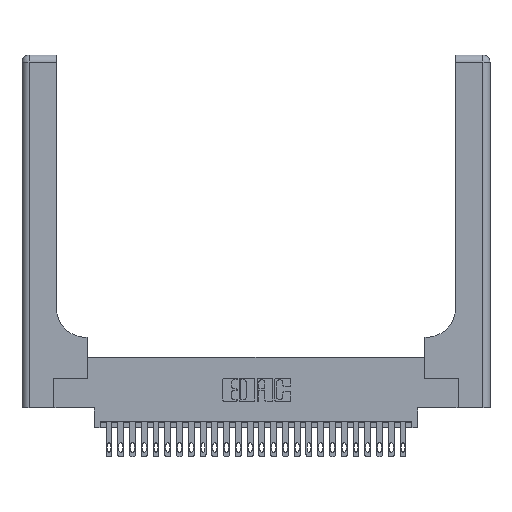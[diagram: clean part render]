
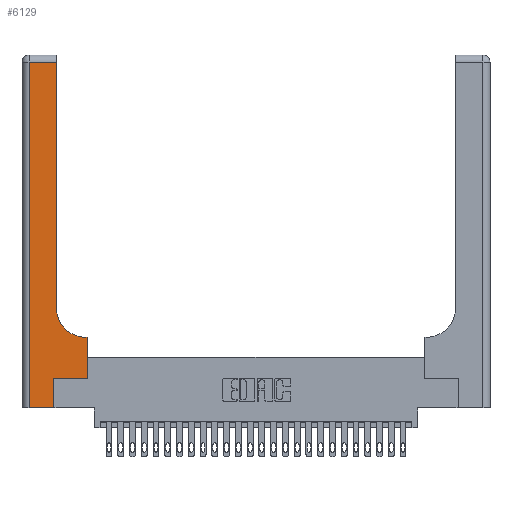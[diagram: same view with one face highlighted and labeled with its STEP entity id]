
A CAD part, top view. The second image highlights one B-rep face of the part: STEP entity #6129.
In plain terms, the highlighted planar face has unit normal (0, 0, 1).
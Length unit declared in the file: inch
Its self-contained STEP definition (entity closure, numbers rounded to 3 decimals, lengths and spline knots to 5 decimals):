
#206 = LINE ( 'NONE', #2875, #23415 ) ;
#1153 = ORIENTED_EDGE ( 'NONE', *, *, #12919, .T. ) ;
#1300 = DIRECTION ( 'NONE',  ( 0., 1., 0. ) ) ;
#1729 = CARTESIAN_POINT ( 'NONE',  ( 0.5585, 0.25, 0.37 ) ) ;
#2001 = CARTESIAN_POINT ( 'NONE',  ( 0.06, 0., 0.37 ) ) ;
#2509 = VERTEX_POINT ( 'NONE', #13331 ) ;
#2572 = LINE ( 'NONE', #18681, #14012 ) ;
#2723 = DIRECTION ( 'NONE',  ( 1., 0., 0. ) ) ;
#2875 = CARTESIAN_POINT ( 'NONE',  ( 0.2915, 3., 0.37 ) ) ;
#3445 = VERTEX_POINT ( 'NONE', #1729 ) ;
#3664 = VERTEX_POINT ( 'NONE', #20395 ) ;
#3770 = VERTEX_POINT ( 'NONE', #18522 ) ;
#4890 = DIRECTION ( 'NONE',  ( -1., 0., 0. ) ) ;
#5336 = EDGE_CURVE ( 'NONE', #13133, #3445, #2572, .T. ) ;
#5775 = EDGE_CURVE ( 'NONE', #22903, #21329, #206, .T. ) ;
#6126 = CARTESIAN_POINT ( 'NONE',  ( 0.2915, 0.6, 0.37 ) ) ;
#6129 = ADVANCED_FACE ( 'NONE', ( #10603 ), #26612, .F. ) ;
#6172 = EDGE_CURVE ( 'NONE', #3664, #22903, #14320, .T. ) ;
#6247 = EDGE_CURVE ( 'NONE', #21329, #3770, #11279, .T. ) ;
#6264 = DIRECTION ( 'NONE',  ( 1., 0., 0. ) ) ;
#6644 = DIRECTION ( 'NONE',  ( 0., -1., 0. ) ) ;
#6783 = LINE ( 'NONE', #12752, #20249 ) ;
#7349 = ORIENTED_EDGE ( 'NONE', *, *, #21374, .T. ) ;
#7609 = AXIS2_PLACEMENT_3D ( 'NONE', #15793, #13718, #2723 ) ;
#8095 = VECTOR ( 'NONE', #6264, 39.37008 ) ;
#8389 = CARTESIAN_POINT ( 'NONE',  ( 0.269, 0.25, 0.37 ) ) ;
#9195 = LINE ( 'NONE', #12284, #16969 ) ;
#9282 = DIRECTION ( 'NONE',  ( 0., 0., -1. ) ) ;
#9646 = ORIENTED_EDGE ( 'NONE', *, *, #5775, .T. ) ;
#10028 = ORIENTED_EDGE ( 'NONE', *, *, #19236, .T. ) ;
#10079 = EDGE_LOOP ( 'NONE', ( #9646, #27332, #13365, #10028, #1153, #11201, #26944, #7349, #20154 ) ) ;
#10603 = FACE_OUTER_BOUND ( 'NONE', #10079, .T. ) ;
#11201 = ORIENTED_EDGE ( 'NONE', *, *, #5336, .T. ) ;
#11279 = LINE ( 'NONE', #13336, #25764 ) ;
#12284 = CARTESIAN_POINT ( 'NONE',  ( 0.5585, 0.25, 0.37 ) ) ;
#12652 = DIRECTION ( 'NONE',  ( 0., 1., 0. ) ) ;
#12752 = CARTESIAN_POINT ( 'NONE',  ( 0.06, 3., 0.37 ) ) ;
#12919 = EDGE_CURVE ( 'NONE', #16148, #13133, #25143, .T. ) ;
#13133 = VERTEX_POINT ( 'NONE', #8389 ) ;
#13331 = CARTESIAN_POINT ( 'NONE',  ( 0.5585, 0.6, 0.37 ) ) ;
#13336 = CARTESIAN_POINT ( 'NONE',  ( 0., 2.94, 0.37 ) ) ;
#13365 = ORIENTED_EDGE ( 'NONE', *, *, #18548, .T. ) ;
#13718 = DIRECTION ( 'NONE',  ( 0., 0., -1. ) ) ;
#14012 = VECTOR ( 'NONE', #20826, 39.37008 ) ;
#14320 = CIRCLE ( 'NONE', #7609, 0.25 ) ;
#15793 = CARTESIAN_POINT ( 'NONE',  ( 0.5415, 0.85, 0.37 ) ) ;
#16010 = VERTEX_POINT ( 'NONE', #2001 ) ;
#16066 = VECTOR ( 'NONE', #1300, 39.37008 ) ;
#16148 = VERTEX_POINT ( 'NONE', #21790 ) ;
#16337 = DIRECTION ( 'NONE',  ( -1., 0., 0. ) ) ;
#16969 = VECTOR ( 'NONE', #12652, 39.37008 ) ;
#18301 = CARTESIAN_POINT ( 'NONE',  ( 0.269, 0., 0.37 ) ) ;
#18522 = CARTESIAN_POINT ( 'NONE',  ( 0.06, 2.94, 0.37 ) ) ;
#18548 = EDGE_CURVE ( 'NONE', #3770, #16010, #6783, .T. ) ;
#18681 = CARTESIAN_POINT ( 'NONE',  ( 0.269, 0.25, 0.37 ) ) ;
#18756 = VECTOR ( 'NONE', #23121, 39.37008 ) ;
#18763 = DIRECTION ( 'NONE',  ( 0., 1., 0. ) ) ;
#18776 = AXIS2_PLACEMENT_3D ( 'NONE', #22269, #9282, #4890 ) ;
#19236 = EDGE_CURVE ( 'NONE', #16010, #16148, #25930, .T. ) ;
#19456 = CARTESIAN_POINT ( 'NONE',  ( 0.2915, 0.85, 0.37 ) ) ;
#20154 = ORIENTED_EDGE ( 'NONE', *, *, #6172, .T. ) ;
#20249 = VECTOR ( 'NONE', #6644, 39.37008 ) ;
#20395 = CARTESIAN_POINT ( 'NONE',  ( 0.5415, 0.6, 0.37 ) ) ;
#20826 = DIRECTION ( 'NONE',  ( 1., 0., 0. ) ) ;
#21108 = CARTESIAN_POINT ( 'NONE',  ( 0., 0., 0.37 ) ) ;
#21329 = VERTEX_POINT ( 'NONE', #23036 ) ;
#21374 = EDGE_CURVE ( 'NONE', #2509, #3664, #24485, .T. ) ;
#21790 = CARTESIAN_POINT ( 'NONE',  ( 0.269, 0., 0.37 ) ) ;
#22269 = CARTESIAN_POINT ( 'NONE',  ( 0., 3., 0.37 ) ) ;
#22903 = VERTEX_POINT ( 'NONE', #19456 ) ;
#23036 = CARTESIAN_POINT ( 'NONE',  ( 0.2915, 2.94, 0.37 ) ) ;
#23121 = DIRECTION ( 'NONE',  ( -1., 0., 0. ) ) ;
#23415 = VECTOR ( 'NONE', #18763, 39.37008 ) ;
#23875 = EDGE_CURVE ( 'NONE', #3445, #2509, #9195, .T. ) ;
#24485 = LINE ( 'NONE', #6126, #18756 ) ;
#25143 = LINE ( 'NONE', #18301, #16066 ) ;
#25764 = VECTOR ( 'NONE', #16337, 39.37008 ) ;
#25930 = LINE ( 'NONE', #21108, #8095 ) ;
#26612 = PLANE ( 'NONE',  #18776 ) ;
#26944 = ORIENTED_EDGE ( 'NONE', *, *, #23875, .T. ) ;
#27332 = ORIENTED_EDGE ( 'NONE', *, *, #6247, .T. ) ;
